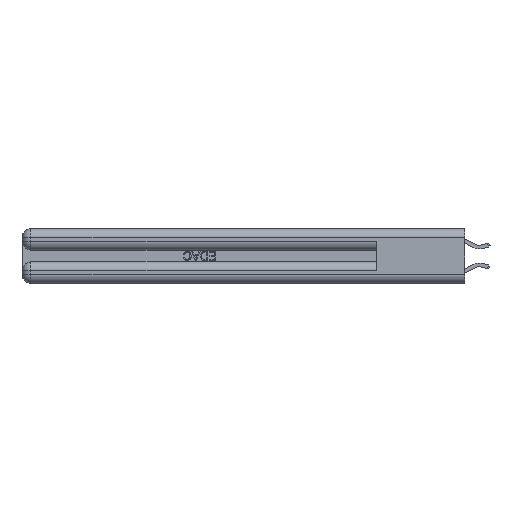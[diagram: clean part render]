
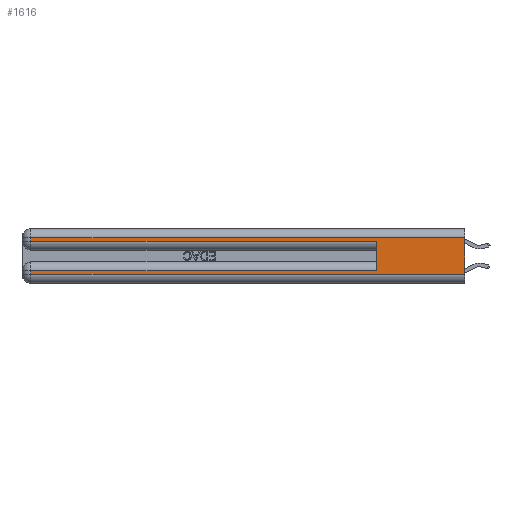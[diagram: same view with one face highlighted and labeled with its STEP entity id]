
A CAD part, left-side view. The second image highlights one B-rep face of the part: STEP entity #1616.
In plain terms, the highlighted planar face has unit normal (-1, 0, 0).
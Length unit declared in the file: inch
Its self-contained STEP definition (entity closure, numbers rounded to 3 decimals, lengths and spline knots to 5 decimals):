
#6 = VECTOR ( 'NONE', #22633, 39.37008 ) ;
#151 = DIRECTION ( 'NONE',  ( 0., 1., 0. ) ) ;
#164 = ORIENTED_EDGE ( 'NONE', *, *, #10040, .T. ) ;
#257 = DIRECTION ( 'NONE',  ( 0., 0., -1. ) ) ;
#393 = EDGE_LOOP ( 'NONE', ( #5247, #13545, #29445, #1477, #11757, #164, #30829, #15386 ) ) ;
#395 = DIRECTION ( 'NONE',  ( 0., -1., 0. ) ) ;
#1477 = ORIENTED_EDGE ( 'NONE', *, *, #2198, .T. ) ;
#1616 = ADVANCED_FACE ( 'NONE', ( #27361 ), #19556, .F. ) ;
#1671 = DIRECTION ( 'NONE',  ( 1., 0., 0. ) ) ;
#2198 = EDGE_CURVE ( 'NONE', #32418, #15011, #23348, .T. ) ;
#2280 = VERTEX_POINT ( 'NONE', #29476 ) ;
#2361 = VECTOR ( 'NONE', #257, 39.37008 ) ;
#3057 = DIRECTION ( 'NONE',  ( 0., 0., -1. ) ) ;
#3522 = CARTESIAN_POINT ( 'NONE',  ( 0., 2.94, 0.31 ) ) ;
#3983 = CARTESIAN_POINT ( 'NONE',  ( 0., 0., 0.37 ) ) ;
#4337 = EDGE_CURVE ( 'NONE', #12258, #32418, #23607, .T. ) ;
#4760 = LINE ( 'NONE', #14835, #6 ) ;
#5057 = CARTESIAN_POINT ( 'NONE',  ( 0., 0.6, 0.145 ) ) ;
#5247 = ORIENTED_EDGE ( 'NONE', *, *, #18536, .F. ) ;
#6925 = EDGE_CURVE ( 'NONE', #19893, #12258, #12726, .T. ) ;
#7127 = EDGE_CURVE ( 'NONE', #2280, #15011, #30249, .T. ) ;
#7390 = EDGE_CURVE ( 'NONE', #31696, #32314, #15473, .T. ) ;
#7400 = VECTOR ( 'NONE', #23655, 39.37008 ) ;
#7712 = CARTESIAN_POINT ( 'NONE',  ( 0., 0., 0.37 ) ) ;
#8957 = CARTESIAN_POINT ( 'NONE',  ( 0., 2.94, 0.06 ) ) ;
#9697 = DIRECTION ( 'NONE',  ( 0., 0., 1. ) ) ;
#9910 = EDGE_CURVE ( 'NONE', #14802, #31696, #31952, .T. ) ;
#10040 = EDGE_CURVE ( 'NONE', #2280, #14802, #4760, .T. ) ;
#11757 = ORIENTED_EDGE ( 'NONE', *, *, #7127, .F. ) ;
#12258 = VERTEX_POINT ( 'NONE', #3522 ) ;
#12726 = LINE ( 'NONE', #22857, #17093 ) ;
#13379 = CARTESIAN_POINT ( 'NONE',  ( 0., 0., 0.285 ) ) ;
#13545 = ORIENTED_EDGE ( 'NONE', *, *, #6925, .T. ) ;
#14802 = VERTEX_POINT ( 'NONE', #20603 ) ;
#14835 = CARTESIAN_POINT ( 'NONE',  ( 0., 0., 0.085 ) ) ;
#15011 = VERTEX_POINT ( 'NONE', #17080 ) ;
#15386 = ORIENTED_EDGE ( 'NONE', *, *, #7390, .T. ) ;
#15473 = LINE ( 'NONE', #25606, #15804 ) ;
#15804 = VECTOR ( 'NONE', #395, 39.37008 ) ;
#16134 = CARTESIAN_POINT ( 'NONE',  ( 0., 2.94, 0.37 ) ) ;
#17080 = CARTESIAN_POINT ( 'NONE',  ( 0., 0.6, 0.285 ) ) ;
#17093 = VECTOR ( 'NONE', #151, 39.37008 ) ;
#17360 = VECTOR ( 'NONE', #18547, 39.37008 ) ;
#17727 = VECTOR ( 'NONE', #9697, 39.37008 ) ;
#17809 = CARTESIAN_POINT ( 'NONE',  ( 0., 0., 0.31 ) ) ;
#18536 = EDGE_CURVE ( 'NONE', #19893, #32314, #28118, .T. ) ;
#18547 = DIRECTION ( 'NONE',  ( 0., -1., 0. ) ) ;
#19556 = PLANE ( 'NONE',  #22229 ) ;
#19893 = VERTEX_POINT ( 'NONE', #17809 ) ;
#20603 = CARTESIAN_POINT ( 'NONE',  ( 0., 2.94, 0.085 ) ) ;
#21003 = CARTESIAN_POINT ( 'NONE',  ( 0., 2.94, 0.285 ) ) ;
#21880 = DIRECTION ( 'NONE',  ( 0., 0., -1. ) ) ;
#22229 = AXIS2_PLACEMENT_3D ( 'NONE', #3983, #1671, #21880 ) ;
#22633 = DIRECTION ( 'NONE',  ( 0., 1., 0. ) ) ;
#22857 = CARTESIAN_POINT ( 'NONE',  ( 0., 0., 0.31 ) ) ;
#23348 = LINE ( 'NONE', #13379, #17360 ) ;
#23607 = LINE ( 'NONE', #16134, #28035 ) ;
#23655 = DIRECTION ( 'NONE',  ( 0., 0., -1. ) ) ;
#24976 = CARTESIAN_POINT ( 'NONE',  ( 0., 0., 0.06 ) ) ;
#25606 = CARTESIAN_POINT ( 'NONE',  ( 0., 0., 0.06 ) ) ;
#26817 = CARTESIAN_POINT ( 'NONE',  ( 0., 2.94, 0.37 ) ) ;
#27361 = FACE_OUTER_BOUND ( 'NONE', #393, .T. ) ;
#28035 = VECTOR ( 'NONE', #3057, 39.37008 ) ;
#28118 = LINE ( 'NONE', #7712, #2361 ) ;
#29445 = ORIENTED_EDGE ( 'NONE', *, *, #4337, .T. ) ;
#29476 = CARTESIAN_POINT ( 'NONE',  ( 0., 0.6, 0.085 ) ) ;
#30249 = LINE ( 'NONE', #5057, #17727 ) ;
#30829 = ORIENTED_EDGE ( 'NONE', *, *, #9910, .T. ) ;
#31696 = VERTEX_POINT ( 'NONE', #8957 ) ;
#31952 = LINE ( 'NONE', #26817, #7400 ) ;
#32314 = VERTEX_POINT ( 'NONE', #24976 ) ;
#32418 = VERTEX_POINT ( 'NONE', #21003 ) ;
